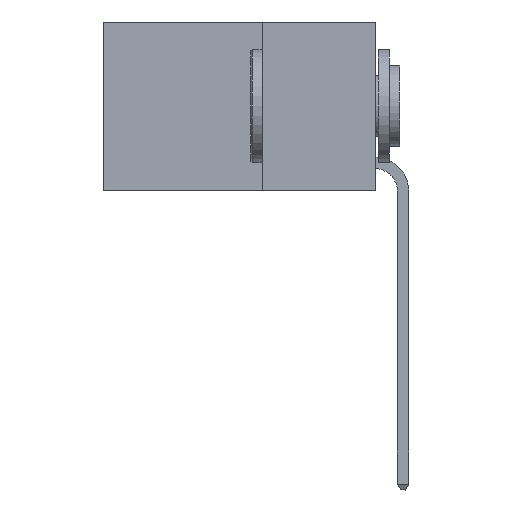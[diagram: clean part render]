
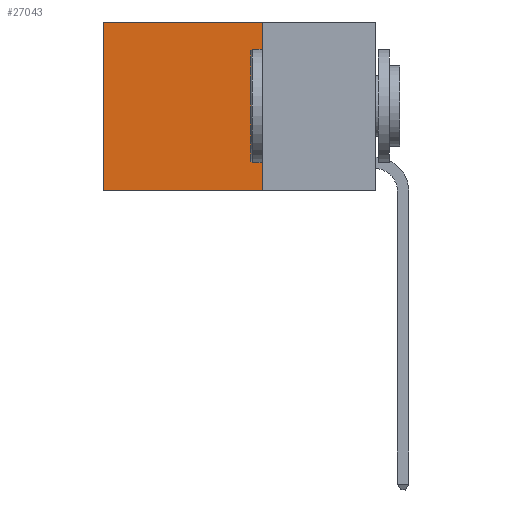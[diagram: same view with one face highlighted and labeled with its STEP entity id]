
A CAD part, left-side view. The second image highlights one B-rep face of the part: STEP entity #27043.
In plain terms, the highlighted planar face has unit normal (-1, 0, 0).
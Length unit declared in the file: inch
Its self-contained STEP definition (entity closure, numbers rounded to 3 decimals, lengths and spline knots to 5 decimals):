
#116 = LINE ( 'NONE', #11145, #16465 ) ;
#1876 = ORIENTED_EDGE ( 'NONE', *, *, #7225, .F. ) ;
#2453 = CARTESIAN_POINT ( 'NONE',  ( 0.2625, 0.25, 0. ) ) ;
#3530 = ORIENTED_EDGE ( 'NONE', *, *, #18240, .F. ) ;
#3755 = LINE ( 'NONE', #8693, #19910 ) ;
#4402 = CARTESIAN_POINT ( 'NONE',  ( 0.2625, 0.6, -0.37 ) ) ;
#4662 = DIRECTION ( 'NONE',  ( 0., 0., -1. ) ) ;
#5515 = VECTOR ( 'NONE', #18525, 39.37008 ) ;
#5906 = VERTEX_POINT ( 'NONE', #14366 ) ;
#7225 = EDGE_CURVE ( 'NONE', #9208, #26616, #16740, .T. ) ;
#7469 = VERTEX_POINT ( 'NONE', #4402 ) ;
#7604 = EDGE_CURVE ( 'NONE', #5906, #7469, #22547, .T. ) ;
#8693 = CARTESIAN_POINT ( 'NONE',  ( 0.2625, 0.25, -0.37 ) ) ;
#9208 = VERTEX_POINT ( 'NONE', #18238 ) ;
#11145 = CARTESIAN_POINT ( 'NONE',  ( 0.2625, 0.25, 0. ) ) ;
#13737 = ORIENTED_EDGE ( 'NONE', *, *, #7604, .T. ) ;
#14366 = CARTESIAN_POINT ( 'NONE',  ( 0.2625, 0.6, 0. ) ) ;
#15262 = CARTESIAN_POINT ( 'NONE',  ( 0.2625, 0.6, 0. ) ) ;
#15694 = AXIS2_PLACEMENT_3D ( 'NONE', #2453, #17292, #4662 ) ;
#16465 = VECTOR ( 'NONE', #17516, 39.37008 ) ;
#16740 = LINE ( 'NONE', #24689, #5515 ) ;
#17018 = VECTOR ( 'NONE', #23747, 39.37008 ) ;
#17292 = DIRECTION ( 'NONE',  ( 1., 0., 0. ) ) ;
#17516 = DIRECTION ( 'NONE',  ( 0., 1., 0. ) ) ;
#18238 = CARTESIAN_POINT ( 'NONE',  ( 0.2625, 0.25, 0. ) ) ;
#18240 = EDGE_CURVE ( 'NONE', #26616, #7469, #3755, .T. ) ;
#18525 = DIRECTION ( 'NONE',  ( 0., 0., -1. ) ) ;
#18805 = FACE_OUTER_BOUND ( 'NONE', #19154, .T. ) ;
#19154 = EDGE_LOOP ( 'NONE', ( #13737, #3530, #1876, #23656 ) ) ;
#19910 = VECTOR ( 'NONE', #21232, 39.37008 ) ;
#21232 = DIRECTION ( 'NONE',  ( 0., 1., 0. ) ) ;
#21351 = EDGE_CURVE ( 'NONE', #9208, #5906, #116, .T. ) ;
#22547 = LINE ( 'NONE', #15262, #17018 ) ;
#23656 = ORIENTED_EDGE ( 'NONE', *, *, #21351, .T. ) ;
#23747 = DIRECTION ( 'NONE',  ( 0., 0., -1. ) ) ;
#24689 = CARTESIAN_POINT ( 'NONE',  ( 0.2625, 0.25, 0. ) ) ;
#25528 = PLANE ( 'NONE',  #15694 ) ;
#26117 = CARTESIAN_POINT ( 'NONE',  ( 0.2625, 0.25, -0.37 ) ) ;
#26616 = VERTEX_POINT ( 'NONE', #26117 ) ;
#27043 = ADVANCED_FACE ( 'NONE', ( #18805 ), #25528, .F. ) ;
